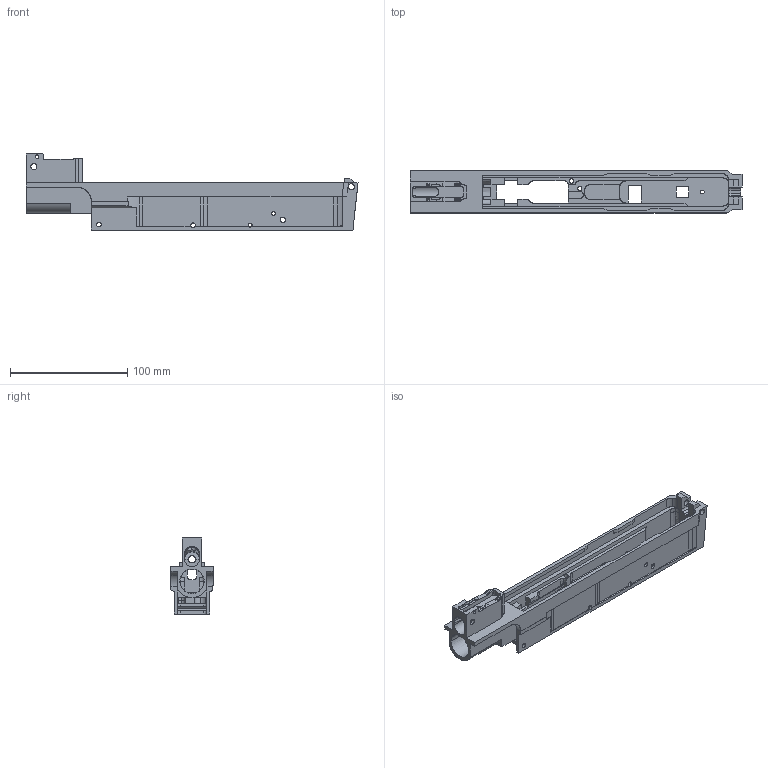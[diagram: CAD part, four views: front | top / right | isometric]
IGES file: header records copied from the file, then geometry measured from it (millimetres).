
Start section: VZ58 Semi By Helix60
Global section: file name: T.MC8; native system: MASTERCAM; preprocessor: 1; date: 071227.051052; units: inch
Bounding box: 283.36 x 35.86 x 64.9 mm (x, y, z)
Surface area: 70593.7 mm2 (no closed solid volume)
Topology: 0 solids, 0 shells, 432 faces, 26043 edges, 27337 vertices
Faces by surface type: bspline 432
